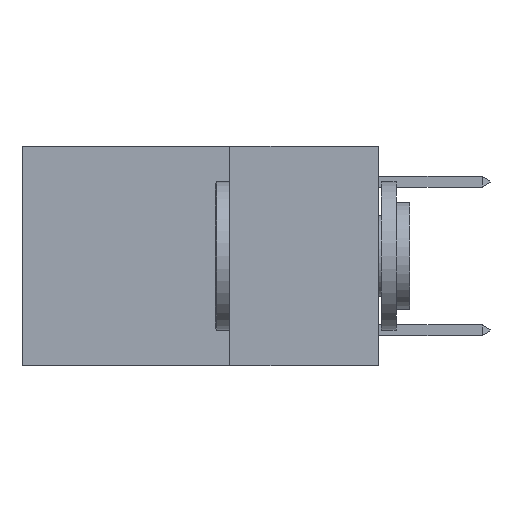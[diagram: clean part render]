
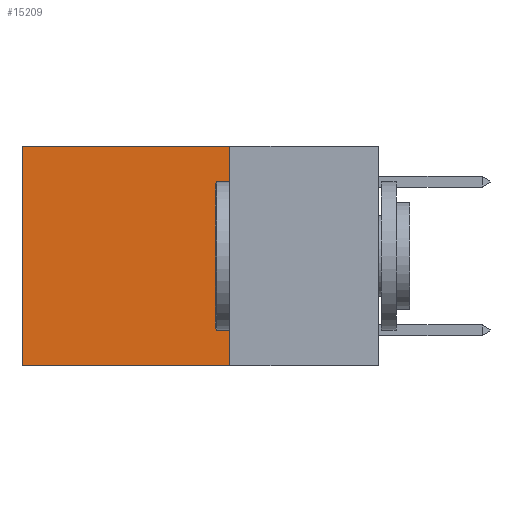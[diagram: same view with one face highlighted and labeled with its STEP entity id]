
A CAD part, left-side view. The second image highlights one B-rep face of the part: STEP entity #15209.
In plain terms, the highlighted planar face has unit normal (-1, 0, 0).
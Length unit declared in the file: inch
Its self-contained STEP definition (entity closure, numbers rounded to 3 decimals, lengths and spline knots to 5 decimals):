
#728 = DIRECTION ( 'NONE',  ( 0., 0., -1. ) ) ;
#1028 = LINE ( 'NONE', #7476, #2638 ) ;
#1037 = FACE_OUTER_BOUND ( 'NONE', #12826, .T. ) ;
#1150 = EDGE_CURVE ( 'NONE', #4948, #17502, #1028, .T. ) ;
#1532 = DIRECTION ( 'NONE',  ( 0., 1., 0. ) ) ;
#2315 = EDGE_CURVE ( 'NONE', #17502, #15185, #10650, .T. ) ;
#2339 = ORIENTED_EDGE ( 'NONE', *, *, #1150, .T. ) ;
#2638 = VECTOR ( 'NONE', #14005, 39.37008 ) ;
#2842 = DIRECTION ( 'NONE',  ( 0., 0., -1. ) ) ;
#2954 = VECTOR ( 'NONE', #1532, 39.37008 ) ;
#3068 = EDGE_CURVE ( 'NONE', #4948, #4242, #5831, .T. ) ;
#3441 = ORIENTED_EDGE ( 'NONE', *, *, #3068, .F. ) ;
#4242 = VERTEX_POINT ( 'NONE', #6877 ) ;
#4796 = ORIENTED_EDGE ( 'NONE', *, *, #9007, .F. ) ;
#4948 = VERTEX_POINT ( 'NONE', #12018 ) ;
#5814 = CARTESIAN_POINT ( 'NONE',  ( 0.2625, 0.25, 0. ) ) ;
#5831 = LINE ( 'NONE', #12153, #20736 ) ;
#6608 = VECTOR ( 'NONE', #17056, 39.37008 ) ;
#6877 = CARTESIAN_POINT ( 'NONE',  ( 0.2625, 0.25, -0.37 ) ) ;
#7476 = CARTESIAN_POINT ( 'NONE',  ( 0.2625, 0.25, 0. ) ) ;
#9007 = EDGE_CURVE ( 'NONE', #4242, #15185, #18833, .T. ) ;
#9416 = AXIS2_PLACEMENT_3D ( 'NONE', #5814, #20237, #2842 ) ;
#10650 = LINE ( 'NONE', #18442, #6608 ) ;
#12018 = CARTESIAN_POINT ( 'NONE',  ( 0.2625, 0.25, 0. ) ) ;
#12153 = CARTESIAN_POINT ( 'NONE',  ( 0.2625, 0.25, 0. ) ) ;
#12424 = CARTESIAN_POINT ( 'NONE',  ( 0.2625, 0.25, -0.37 ) ) ;
#12826 = EDGE_LOOP ( 'NONE', ( #13663, #4796, #3441, #2339 ) ) ;
#13663 = ORIENTED_EDGE ( 'NONE', *, *, #2315, .T. ) ;
#14005 = DIRECTION ( 'NONE',  ( 0., 1., 0. ) ) ;
#14126 = PLANE ( 'NONE',  #9416 ) ;
#15185 = VERTEX_POINT ( 'NONE', #15694 ) ;
#15209 = ADVANCED_FACE ( 'NONE', ( #1037 ), #14126, .F. ) ;
#15694 = CARTESIAN_POINT ( 'NONE',  ( 0.2625, 0.6, -0.37 ) ) ;
#17056 = DIRECTION ( 'NONE',  ( 0., 0., -1. ) ) ;
#17502 = VERTEX_POINT ( 'NONE', #20179 ) ;
#18442 = CARTESIAN_POINT ( 'NONE',  ( 0.2625, 0.6, 0. ) ) ;
#18833 = LINE ( 'NONE', #12424, #2954 ) ;
#20179 = CARTESIAN_POINT ( 'NONE',  ( 0.2625, 0.6, 0. ) ) ;
#20237 = DIRECTION ( 'NONE',  ( 1., 0., 0. ) ) ;
#20736 = VECTOR ( 'NONE', #728, 39.37008 ) ;
